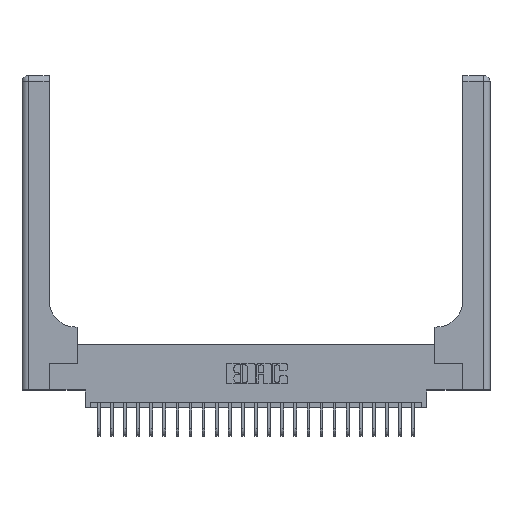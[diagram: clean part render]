
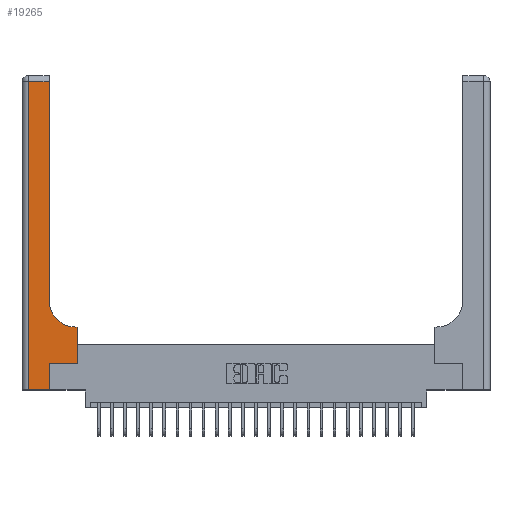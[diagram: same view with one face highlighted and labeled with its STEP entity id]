
A CAD part, top view. The second image highlights one B-rep face of the part: STEP entity #19265.
In plain terms, the highlighted planar face has unit normal (0, 0, 1).
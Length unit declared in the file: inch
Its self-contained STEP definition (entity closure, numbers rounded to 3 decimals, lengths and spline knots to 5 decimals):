
#26 = LINE ( 'NONE', #15780, #11566 ) ;
#56 = CARTESIAN_POINT ( 'NONE',  ( 0.26, 3., 0.37 ) ) ;
#145 = ORIENTED_EDGE ( 'NONE', *, *, #3469, .T. ) ;
#464 = EDGE_CURVE ( 'NONE', #19828, #2094, #3004, .T. ) ;
#1026 = VECTOR ( 'NONE', #7208, 39.37008 ) ;
#1039 = ORIENTED_EDGE ( 'NONE', *, *, #16799, .T. ) ;
#1202 = CARTESIAN_POINT ( 'NONE',  ( 0.265, 0., 0.37 ) ) ;
#2094 = VERTEX_POINT ( 'NONE', #22713 ) ;
#2199 = DIRECTION ( 'NONE',  ( -1., 0., 0. ) ) ;
#2511 = DIRECTION ( 'NONE',  ( -1., 0., 0. ) ) ;
#2951 = CARTESIAN_POINT ( 'NONE',  ( 0.06, 2.94, 0.37 ) ) ;
#3004 = LINE ( 'NONE', #25249, #23177 ) ;
#3469 = EDGE_CURVE ( 'NONE', #9911, #18504, #9201, .T. ) ;
#3731 = ORIENTED_EDGE ( 'NONE', *, *, #15176, .T. ) ;
#4496 = CARTESIAN_POINT ( 'NONE',  ( 0., 2.94, 0.37 ) ) ;
#4572 = EDGE_LOOP ( 'NONE', ( #5198, #5890, #7760, #1039, #13900, #3731, #9598, #145, #22514 ) ) ;
#5142 = VERTEX_POINT ( 'NONE', #9061 ) ;
#5198 = ORIENTED_EDGE ( 'NONE', *, *, #14655, .T. ) ;
#5890 = ORIENTED_EDGE ( 'NONE', *, *, #6940, .T. ) ;
#6039 = VECTOR ( 'NONE', #24291, 39.37008 ) ;
#6730 = LINE ( 'NONE', #4496, #13580 ) ;
#6940 = EDGE_CURVE ( 'NONE', #18236, #19828, #6730, .T. ) ;
#7208 = DIRECTION ( 'NONE',  ( -1., 0., 0. ) ) ;
#7548 = DIRECTION ( 'NONE',  ( 0., 0., -1. ) ) ;
#7760 = ORIENTED_EDGE ( 'NONE', *, *, #464, .T. ) ;
#9061 = CARTESIAN_POINT ( 'NONE',  ( 0.528, 0.25, 0.37 ) ) ;
#9187 = CARTESIAN_POINT ( 'NONE',  ( 0.51, 0.6, 0.37 ) ) ;
#9201 = LINE ( 'NONE', #25364, #1026 ) ;
#9444 = VECTOR ( 'NONE', #13352, 39.37008 ) ;
#9598 = ORIENTED_EDGE ( 'NONE', *, *, #15004, .T. ) ;
#9780 = VERTEX_POINT ( 'NONE', #25593 ) ;
#9911 = VERTEX_POINT ( 'NONE', #26096 ) ;
#10237 = VERTEX_POINT ( 'NONE', #1202 ) ;
#10364 = LINE ( 'NONE', #18436, #21725 ) ;
#10615 = AXIS2_PLACEMENT_3D ( 'NONE', #20186, #18065, #2199 ) ;
#11113 = VERTEX_POINT ( 'NONE', #19276 ) ;
#11566 = VECTOR ( 'NONE', #20264, 39.37008 ) ;
#11615 = CARTESIAN_POINT ( 'NONE',  ( 0.265, 0.25, 0.37 ) ) ;
#13129 = AXIS2_PLACEMENT_3D ( 'NONE', #19743, #7548, #13780 ) ;
#13352 = DIRECTION ( 'NONE',  ( 1., 0., 0. ) ) ;
#13580 = VECTOR ( 'NONE', #2511, 39.37008 ) ;
#13780 = DIRECTION ( 'NONE',  ( 1., 0., 0. ) ) ;
#13900 = ORIENTED_EDGE ( 'NONE', *, *, #17370, .T. ) ;
#14655 = EDGE_CURVE ( 'NONE', #11113, #18236, #20052, .T. ) ;
#15004 = EDGE_CURVE ( 'NONE', #5142, #9911, #26, .T. ) ;
#15176 = EDGE_CURVE ( 'NONE', #9780, #5142, #23799, .T. ) ;
#15339 = LINE ( 'NONE', #23430, #9444 ) ;
#15780 = CARTESIAN_POINT ( 'NONE',  ( 0.528, 0.25, 0.37 ) ) ;
#15792 = DIRECTION ( 'NONE',  ( 0., 1., 0. ) ) ;
#16741 = CARTESIAN_POINT ( 'NONE',  ( 0.26, 2.94, 0.37 ) ) ;
#16799 = EDGE_CURVE ( 'NONE', #2094, #10237, #15339, .T. ) ;
#17370 = EDGE_CURVE ( 'NONE', #10237, #9780, #10364, .T. ) ;
#17570 = DIRECTION ( 'NONE',  ( 1., 0., 0. ) ) ;
#18065 = DIRECTION ( 'NONE',  ( 0., 0., -1. ) ) ;
#18236 = VERTEX_POINT ( 'NONE', #16741 ) ;
#18436 = CARTESIAN_POINT ( 'NONE',  ( 0.265, 0., 0.37 ) ) ;
#18504 = VERTEX_POINT ( 'NONE', #9187 ) ;
#19265 = ADVANCED_FACE ( 'NONE', ( #24571 ), #24718, .F. ) ;
#19276 = CARTESIAN_POINT ( 'NONE',  ( 0.26, 0.85, 0.37 ) ) ;
#19743 = CARTESIAN_POINT ( 'NONE',  ( 0.51, 0.85, 0.37 ) ) ;
#19828 = VERTEX_POINT ( 'NONE', #2951 ) ;
#20052 = LINE ( 'NONE', #56, #6039 ) ;
#20058 = EDGE_CURVE ( 'NONE', #18504, #11113, #25400, .T. ) ;
#20186 = CARTESIAN_POINT ( 'NONE',  ( 0., 3., 0.37 ) ) ;
#20264 = DIRECTION ( 'NONE',  ( 0., 1., 0. ) ) ;
#20443 = VECTOR ( 'NONE', #17570, 39.37008 ) ;
#21725 = VECTOR ( 'NONE', #15792, 39.37008 ) ;
#22514 = ORIENTED_EDGE ( 'NONE', *, *, #20058, .T. ) ;
#22713 = CARTESIAN_POINT ( 'NONE',  ( 0.06, 0., 0.37 ) ) ;
#23177 = VECTOR ( 'NONE', #23525, 39.37008 ) ;
#23430 = CARTESIAN_POINT ( 'NONE',  ( 0., 0., 0.37 ) ) ;
#23525 = DIRECTION ( 'NONE',  ( 0., -1., 0. ) ) ;
#23799 = LINE ( 'NONE', #11615, #20443 ) ;
#24291 = DIRECTION ( 'NONE',  ( 0., 1., 0. ) ) ;
#24571 = FACE_OUTER_BOUND ( 'NONE', #4572, .T. ) ;
#24718 = PLANE ( 'NONE',  #10615 ) ;
#25249 = CARTESIAN_POINT ( 'NONE',  ( 0.06, 3., 0.37 ) ) ;
#25364 = CARTESIAN_POINT ( 'NONE',  ( 0.26, 0.6, 0.37 ) ) ;
#25400 = CIRCLE ( 'NONE', #13129, 0.25 ) ;
#25593 = CARTESIAN_POINT ( 'NONE',  ( 0.265, 0.25, 0.37 ) ) ;
#26096 = CARTESIAN_POINT ( 'NONE',  ( 0.528, 0.6, 0.37 ) ) ;
